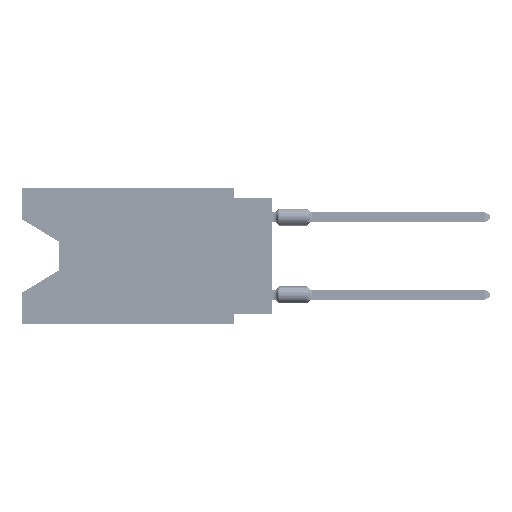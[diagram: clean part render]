
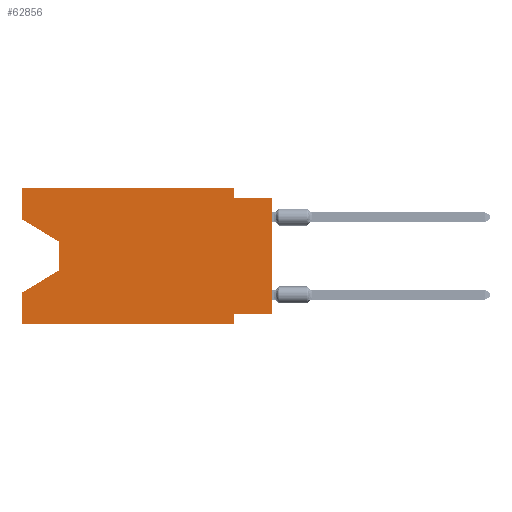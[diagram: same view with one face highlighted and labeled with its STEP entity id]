
A CAD part, left-side view. The second image highlights one B-rep face of the part: STEP entity #62856.
In plain terms, the highlighted planar face has unit normal (-1, 0, 0).
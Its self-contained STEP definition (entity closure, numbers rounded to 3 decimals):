
#467 = ORIENTED_EDGE ( 'NONE', *, *, #21522, .T. ) ;
#854 = CARTESIAN_POINT ( 'NONE',  ( 0., 16.383, 0. ) ) ;
#3022 = CARTESIAN_POINT ( 'NONE',  ( 0., 16.383, -2.038 ) ) ;
#3154 = EDGE_CURVE ( 'NONE', #64855, #64046, #50895, .T. ) ;
#3399 = CARTESIAN_POINT ( 'NONE',  ( 0., 13.97, -5.385 ) ) ;
#5898 = VERTEX_POINT ( 'NONE', #8924 ) ;
#6532 = EDGE_CURVE ( 'NONE', #23465, #9368, #22379, .T. ) ;
#7743 = DIRECTION ( 'NONE',  ( 0., 0., -1. ) ) ;
#7827 = ORIENTED_EDGE ( 'NONE', *, *, #45707, .F. ) ;
#8924 = CARTESIAN_POINT ( 'NONE',  ( 0., 2.54, -0.635 ) ) ;
#9368 = VERTEX_POINT ( 'NONE', #51939 ) ;
#9485 = DIRECTION ( 'NONE',  ( 0., 0.855, -0.519 ) ) ;
#10091 = LINE ( 'NONE', #47677, #11771 ) ;
#10275 = LINE ( 'NONE', #65351, #41882 ) ;
#11090 = FACE_OUTER_BOUND ( 'NONE', #56201, .T. ) ;
#11771 = VECTOR ( 'NONE', #15465, 1000. ) ;
#13113 = LINE ( 'NONE', #13820, #49065 ) ;
#13307 = EDGE_CURVE ( 'NONE', #30723, #22088, #68478, .T. ) ;
#13820 = CARTESIAN_POINT ( 'NONE',  ( 0., 2.54, 0. ) ) ;
#14112 = DIRECTION ( 'NONE',  ( 0., -0.855, -0.519 ) ) ;
#15465 = DIRECTION ( 'NONE',  ( 0., 0., -1. ) ) ;
#15612 = CARTESIAN_POINT ( 'NONE',  ( 0., 16.383, -8.89 ) ) ;
#16874 = CARTESIAN_POINT ( 'NONE',  ( 0., 0., -0.635 ) ) ;
#17675 = EDGE_CURVE ( 'NONE', #20852, #53505, #58507, .T. ) ;
#18961 = DIRECTION ( 'NONE',  ( 0., 0., 1. ) ) ;
#20102 = EDGE_CURVE ( 'NONE', #33363, #20679, #55427, .T. ) ;
#20145 = VECTOR ( 'NONE', #9485, 1000. ) ;
#20679 = VERTEX_POINT ( 'NONE', #24559 ) ;
#20779 = PLANE ( 'NONE',  #59335 ) ;
#20852 = VERTEX_POINT ( 'NONE', #34509 ) ;
#20978 = DIRECTION ( 'NONE',  ( 0., -1., 0. ) ) ;
#21131 = DIRECTION ( 'NONE',  ( 0., 0., -1. ) ) ;
#21522 = EDGE_CURVE ( 'NONE', #22088, #20852, #50851, .T. ) ;
#22088 = VERTEX_POINT ( 'NONE', #62824 ) ;
#22379 = LINE ( 'NONE', #15612, #46560 ) ;
#22489 = ORIENTED_EDGE ( 'NONE', *, *, #17675, .T. ) ;
#23465 = VERTEX_POINT ( 'NONE', #52543 ) ;
#23578 = DIRECTION ( 'NONE',  ( 0., 1., 0. ) ) ;
#24559 = CARTESIAN_POINT ( 'NONE',  ( 0., 2.54, -8.255 ) ) ;
#26173 = VERTEX_POINT ( 'NONE', #16874 ) ;
#28049 = ORIENTED_EDGE ( 'NONE', *, *, #55647, .F. ) ;
#28644 = LINE ( 'NONE', #29717, #55442 ) ;
#29419 = ORIENTED_EDGE ( 'NONE', *, *, #57313, .F. ) ;
#29717 = CARTESIAN_POINT ( 'NONE',  ( 0., 0., -0.635 ) ) ;
#30247 = VECTOR ( 'NONE', #18961, 1000. ) ;
#30723 = VERTEX_POINT ( 'NONE', #64783 ) ;
#32223 = DIRECTION ( 'NONE',  ( 1., 0., 0. ) ) ;
#32282 = ORIENTED_EDGE ( 'NONE', *, *, #67851, .T. ) ;
#33363 = VERTEX_POINT ( 'NONE', #70095 ) ;
#34137 = DIRECTION ( 'NONE',  ( 0., 0., 1. ) ) ;
#34509 = CARTESIAN_POINT ( 'NONE',  ( 0., 13.97, -5.385 ) ) ;
#34892 = ORIENTED_EDGE ( 'NONE', *, *, #20102, .F. ) ;
#35435 = VECTOR ( 'NONE', #40162, 1000. ) ;
#37006 = CARTESIAN_POINT ( 'NONE',  ( 0., 16.383, 0. ) ) ;
#38939 = EDGE_CURVE ( 'NONE', #30723, #64855, #56885, .T. ) ;
#39423 = DIRECTION ( 'NONE',  ( 0., 0., -1. ) ) ;
#40162 = DIRECTION ( 'NONE',  ( 0., -1., 0. ) ) ;
#40195 = VECTOR ( 'NONE', #14112, 1000. ) ;
#41882 = VECTOR ( 'NONE', #34137, 1000. ) ;
#42785 = VECTOR ( 'NONE', #64528, 1000. ) ;
#45707 = EDGE_CURVE ( 'NONE', #5898, #26173, #28644, .T. ) ;
#45881 = CARTESIAN_POINT ( 'NONE',  ( 0., 16.383, 0. ) ) ;
#46192 = CARTESIAN_POINT ( 'NONE',  ( 0., 13.97, -3.505 ) ) ;
#46560 = VECTOR ( 'NONE', #20978, 1000. ) ;
#47258 = ORIENTED_EDGE ( 'NONE', *, *, #6532, .T. ) ;
#47677 = CARTESIAN_POINT ( 'NONE',  ( 0., 2.54, -8.89 ) ) ;
#48075 = LINE ( 'NONE', #37006, #42785 ) ;
#48090 = ORIENTED_EDGE ( 'NONE', *, *, #13307, .T. ) ;
#49065 = VECTOR ( 'NONE', #7743, 1000. ) ;
#49230 = ORIENTED_EDGE ( 'NONE', *, *, #3154, .F. ) ;
#50760 = CARTESIAN_POINT ( 'NONE',  ( 0., 0., -8.255 ) ) ;
#50817 = DIRECTION ( 'NONE',  ( 0., -1., 0. ) ) ;
#50851 = LINE ( 'NONE', #46192, #57133 ) ;
#50895 = LINE ( 'NONE', #45881, #35435 ) ;
#51259 = VECTOR ( 'NONE', #23578, 1000. ) ;
#51403 = CARTESIAN_POINT ( 'NONE',  ( 0., 16.383, -6.852 ) ) ;
#51861 = CARTESIAN_POINT ( 'NONE',  ( 0., 16.383, 0. ) ) ;
#51939 = CARTESIAN_POINT ( 'NONE',  ( 0., 2.54, -8.89 ) ) ;
#52543 = CARTESIAN_POINT ( 'NONE',  ( 0., 16.383, -8.89 ) ) ;
#53505 = VERTEX_POINT ( 'NONE', #51403 ) ;
#55427 = LINE ( 'NONE', #50760, #51259 ) ;
#55442 = VECTOR ( 'NONE', #50817, 1000. ) ;
#55647 = EDGE_CURVE ( 'NONE', #20679, #9368, #10091, .T. ) ;
#56201 = EDGE_LOOP ( 'NONE', ( #48090, #467, #22489, #29419, #47258, #28049, #34892, #32282, #7827, #63727, #49230, #61778 ) ) ;
#56885 = LINE ( 'NONE', #51861, #30247 ) ;
#57133 = VECTOR ( 'NONE', #39423, 1000. ) ;
#57313 = EDGE_CURVE ( 'NONE', #23465, #53505, #48075, .T. ) ;
#58507 = LINE ( 'NONE', #3399, #20145 ) ;
#59335 = AXIS2_PLACEMENT_3D ( 'NONE', #64427, #32223, #21131 ) ;
#61778 = ORIENTED_EDGE ( 'NONE', *, *, #38939, .F. ) ;
#62824 = CARTESIAN_POINT ( 'NONE',  ( 0., 13.97, -3.505 ) ) ;
#62856 = ADVANCED_FACE ( 'NONE', ( #11090 ), #20779, .F. ) ;
#63595 = EDGE_CURVE ( 'NONE', #64046, #5898, #13113, .T. ) ;
#63727 = ORIENTED_EDGE ( 'NONE', *, *, #63595, .F. ) ;
#64046 = VERTEX_POINT ( 'NONE', #67772 ) ;
#64427 = CARTESIAN_POINT ( 'NONE',  ( 0., 16.383, 0. ) ) ;
#64528 = DIRECTION ( 'NONE',  ( 0., 0., 1. ) ) ;
#64783 = CARTESIAN_POINT ( 'NONE',  ( 0., 16.383, -2.038 ) ) ;
#64855 = VERTEX_POINT ( 'NONE', #854 ) ;
#65351 = CARTESIAN_POINT ( 'NONE',  ( 0., 0., 0. ) ) ;
#67772 = CARTESIAN_POINT ( 'NONE',  ( 0., 2.54, 0. ) ) ;
#67851 = EDGE_CURVE ( 'NONE', #33363, #26173, #10275, .T. ) ;
#68478 = LINE ( 'NONE', #3022, #40195 ) ;
#70095 = CARTESIAN_POINT ( 'NONE',  ( 0., 0., -8.255 ) ) ;
